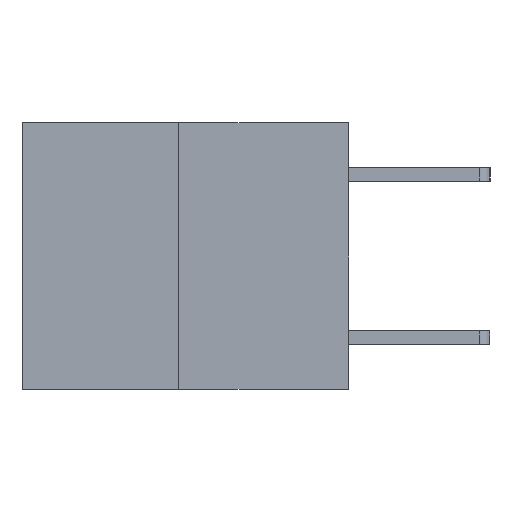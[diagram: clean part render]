
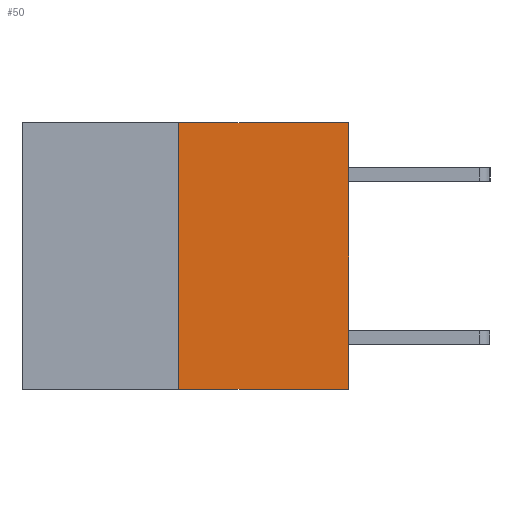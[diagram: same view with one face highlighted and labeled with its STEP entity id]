
A CAD part, left-side view. The second image highlights one B-rep face of the part: STEP entity #50.
In plain terms, the highlighted planar face has unit normal (-1, 0, 0).
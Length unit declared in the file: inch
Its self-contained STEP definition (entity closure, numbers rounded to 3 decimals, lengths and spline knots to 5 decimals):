
#50 = ADVANCED_FACE ( 'NONE', ( #9547 ), #10125, .F. ) ;
#92 = CARTESIAN_POINT ( 'NONE',  ( 0., 0., -0.49 ) ) ;
#243 = VECTOR ( 'NONE', #5901, 39.37008 ) ;
#256 = EDGE_CURVE ( 'NONE', #7647, #8284, #2787, .T. ) ;
#1436 = VECTOR ( 'NONE', #11395, 39.37008 ) ;
#1474 = CARTESIAN_POINT ( 'NONE',  ( 0., 0.6, 0. ) ) ;
#1813 = VECTOR ( 'NONE', #3310, 39.37008 ) ;
#2136 = CARTESIAN_POINT ( 'NONE',  ( 0., 0.312, -0.49 ) ) ;
#2155 = CARTESIAN_POINT ( 'NONE',  ( 0., 0.312, 0. ) ) ;
#2449 = LINE ( 'NONE', #7090, #6989 ) ;
#2541 = VERTEX_POINT ( 'NONE', #2155 ) ;
#2573 = DIRECTION ( 'NONE',  ( 0., 0., 1. ) ) ;
#2787 = LINE ( 'NONE', #8498, #243 ) ;
#2840 = LINE ( 'NONE', #7914, #1436 ) ;
#3310 = DIRECTION ( 'NONE',  ( 0., -1., 0. ) ) ;
#4161 = EDGE_CURVE ( 'NONE', #2541, #8284, #4917, .T. ) ;
#4504 = ORIENTED_EDGE ( 'NONE', *, *, #256, .T. ) ;
#4830 = EDGE_LOOP ( 'NONE', ( #9896, #8594, #4504, #9378 ) ) ;
#4917 = LINE ( 'NONE', #1474, #1813 ) ;
#5901 = DIRECTION ( 'NONE',  ( 0., 0., 1. ) ) ;
#6060 = EDGE_CURVE ( 'NONE', #8989, #2541, #2449, .T. ) ;
#6532 = DIRECTION ( 'NONE',  ( 1., 0., 0. ) ) ;
#6652 = DIRECTION ( 'NONE',  ( 0., 0., -1. ) ) ;
#6667 = CARTESIAN_POINT ( 'NONE',  ( 0., 0., 0. ) ) ;
#6989 = VECTOR ( 'NONE', #2573, 39.37008 ) ;
#7090 = CARTESIAN_POINT ( 'NONE',  ( 0., 0.312, -0.49 ) ) ;
#7647 = VERTEX_POINT ( 'NONE', #92 ) ;
#7914 = CARTESIAN_POINT ( 'NONE',  ( 0., 0.6, -0.49 ) ) ;
#8284 = VERTEX_POINT ( 'NONE', #6667 ) ;
#8498 = CARTESIAN_POINT ( 'NONE',  ( 0., 0., 0. ) ) ;
#8588 = AXIS2_PLACEMENT_3D ( 'NONE', #10164, #6532, #6652 ) ;
#8594 = ORIENTED_EDGE ( 'NONE', *, *, #8702, .T. ) ;
#8702 = EDGE_CURVE ( 'NONE', #8989, #7647, #2840, .T. ) ;
#8989 = VERTEX_POINT ( 'NONE', #2136 ) ;
#9378 = ORIENTED_EDGE ( 'NONE', *, *, #4161, .F. ) ;
#9547 = FACE_OUTER_BOUND ( 'NONE', #4830, .T. ) ;
#9896 = ORIENTED_EDGE ( 'NONE', *, *, #6060, .F. ) ;
#10125 = PLANE ( 'NONE',  #8588 ) ;
#10164 = CARTESIAN_POINT ( 'NONE',  ( 0., 0.6, 0. ) ) ;
#11395 = DIRECTION ( 'NONE',  ( 0., -1., 0. ) ) ;
